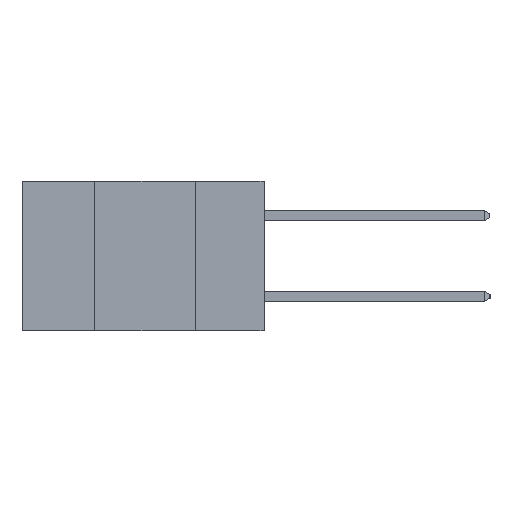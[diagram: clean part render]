
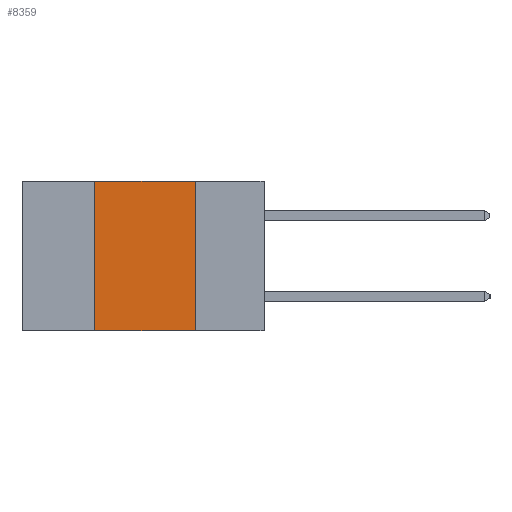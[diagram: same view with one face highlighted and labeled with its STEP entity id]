
A CAD part, left-side view. The second image highlights one B-rep face of the part: STEP entity #8359.
In plain terms, the highlighted planar face has unit normal (-1, 0, 0).
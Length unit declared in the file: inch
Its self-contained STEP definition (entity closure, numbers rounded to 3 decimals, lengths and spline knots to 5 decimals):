
#206 = VERTEX_POINT ( 'NONE', #13072 ) ;
#825 = VECTOR ( 'NONE', #8530, 39.37008 ) ;
#902 = CARTESIAN_POINT ( 'NONE',  ( 0., 0.6, 0. ) ) ;
#1248 = FACE_OUTER_BOUND ( 'NONE', #10583, .T. ) ;
#1602 = VERTEX_POINT ( 'NONE', #5852 ) ;
#1761 = EDGE_CURVE ( 'NONE', #11131, #206, #4994, .T. ) ;
#2130 = PLANE ( 'NONE',  #3319 ) ;
#2725 = VECTOR ( 'NONE', #11576, 39.37008 ) ;
#3319 = AXIS2_PLACEMENT_3D ( 'NONE', #9792, #13630, #5950 ) ;
#3449 = EDGE_CURVE ( 'NONE', #11131, #16231, #5691, .T. ) ;
#3945 = VECTOR ( 'NONE', #10601, 39.37008 ) ;
#4994 = LINE ( 'NONE', #12616, #15247 ) ;
#5691 = LINE ( 'NONE', #10348, #2725 ) ;
#5852 = CARTESIAN_POINT ( 'NONE',  ( 0., 0.17, 0. ) ) ;
#5950 = DIRECTION ( 'NONE',  ( 0., 0., -1. ) ) ;
#6063 = CARTESIAN_POINT ( 'NONE',  ( 0., 0.42, -0.37 ) ) ;
#7181 = ORIENTED_EDGE ( 'NONE', *, *, #11751, .F. ) ;
#8359 = ADVANCED_FACE ( 'NONE', ( #1248 ), #2130, .F. ) ;
#8530 = DIRECTION ( 'NONE',  ( 0., -1., 0. ) ) ;
#9792 = CARTESIAN_POINT ( 'NONE',  ( 0., 0.6, 0. ) ) ;
#10083 = DIRECTION ( 'NONE',  ( 0., 0., 1. ) ) ;
#10175 = CARTESIAN_POINT ( 'NONE',  ( 0., 0.17, -0.37 ) ) ;
#10348 = CARTESIAN_POINT ( 'NONE',  ( 0., 0.6, -0.37 ) ) ;
#10583 = EDGE_LOOP ( 'NONE', ( #12096, #7181, #11736, #13375 ) ) ;
#10601 = DIRECTION ( 'NONE',  ( 0., 0., -1. ) ) ;
#10986 = LINE ( 'NONE', #902, #825 ) ;
#11131 = VERTEX_POINT ( 'NONE', #6063 ) ;
#11558 = EDGE_CURVE ( 'NONE', #1602, #16231, #14592, .T. ) ;
#11576 = DIRECTION ( 'NONE',  ( 0., -1., 0. ) ) ;
#11736 = ORIENTED_EDGE ( 'NONE', *, *, #1761, .F. ) ;
#11751 = EDGE_CURVE ( 'NONE', #206, #1602, #10986, .T. ) ;
#11958 = CARTESIAN_POINT ( 'NONE',  ( 0., 0.17, -0.37 ) ) ;
#12096 = ORIENTED_EDGE ( 'NONE', *, *, #11558, .F. ) ;
#12616 = CARTESIAN_POINT ( 'NONE',  ( 0., 0.42, -0.37 ) ) ;
#13072 = CARTESIAN_POINT ( 'NONE',  ( 0., 0.42, 0. ) ) ;
#13375 = ORIENTED_EDGE ( 'NONE', *, *, #3449, .T. ) ;
#13630 = DIRECTION ( 'NONE',  ( 1., 0., 0. ) ) ;
#14592 = LINE ( 'NONE', #11958, #3945 ) ;
#15247 = VECTOR ( 'NONE', #10083, 39.37008 ) ;
#16231 = VERTEX_POINT ( 'NONE', #10175 ) ;
